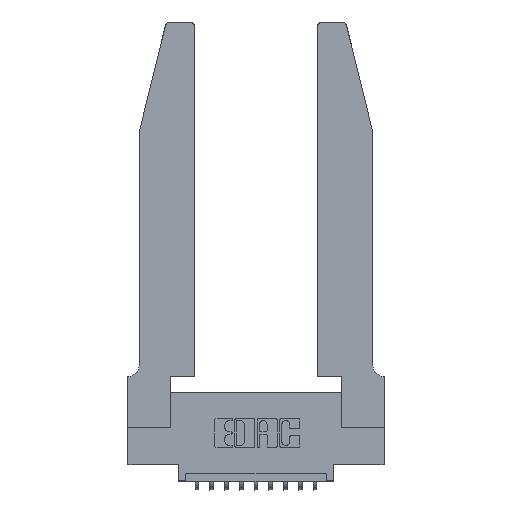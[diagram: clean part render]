
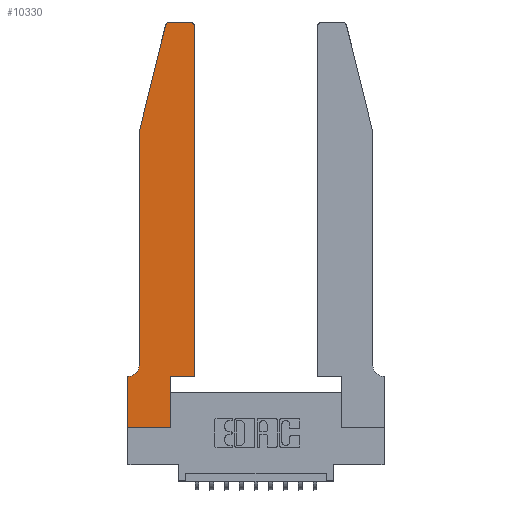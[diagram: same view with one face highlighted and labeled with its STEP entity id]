
A CAD part, top view. The second image highlights one B-rep face of the part: STEP entity #10330.
In plain terms, the highlighted planar face has unit normal (0, 0, 1).
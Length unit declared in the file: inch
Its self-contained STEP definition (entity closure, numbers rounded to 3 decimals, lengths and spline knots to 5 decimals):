
#149 = CARTESIAN_POINT ( 'NONE',  ( 0.25487, 2.72718, 0.37 ) ) ;
#305 = ORIENTED_EDGE ( 'NONE', *, *, #7473, .T. ) ;
#687 = DIRECTION ( 'NONE',  ( 0., 0., -1. ) ) ;
#851 = CARTESIAN_POINT ( 'NONE',  ( 0.4505, 2.72, 0.37 ) ) ;
#984 = EDGE_CURVE ( 'NONE', #15779, #5877, #7594, .T. ) ;
#1242 = ORIENTED_EDGE ( 'NONE', *, *, #15921, .T. ) ;
#1302 = VECTOR ( 'NONE', #8511, 39.37008 ) ;
#1312 = LINE ( 'NONE', #13618, #15610 ) ;
#1523 = CARTESIAN_POINT ( 'NONE',  ( 0.284, 2.72, 0.37 ) ) ;
#1672 = EDGE_CURVE ( 'NONE', #11569, #14212, #6824, .T. ) ;
#1750 = LINE ( 'NONE', #10745, #3556 ) ;
#1878 = CARTESIAN_POINT ( 'NONE',  ( 0.4205, 2.75, 0.37 ) ) ;
#1890 = EDGE_CURVE ( 'NONE', #8346, #9849, #11443, .T. ) ;
#2025 = CARTESIAN_POINT ( 'NONE',  ( 0., 0.35, 0.37 ) ) ;
#2319 = CARTESIAN_POINT ( 'NONE',  ( 0., 0., 0.37 ) ) ;
#2648 = VECTOR ( 'NONE', #5698, 39.37008 ) ;
#2650 = DIRECTION ( 'NONE',  ( 1., 0., 0. ) ) ;
#2751 = CIRCLE ( 'NONE', #11983, 0.07 ) ;
#2765 = DIRECTION ( 'NONE',  ( 0., 0., 1. ) ) ;
#3120 = LINE ( 'NONE', #12759, #15972 ) ;
#3165 = CIRCLE ( 'NONE', #11221, 0.03 ) ;
#3261 = DIRECTION ( 'NONE',  ( 0., 0., 1. ) ) ;
#3475 = CARTESIAN_POINT ( 'NONE',  ( 0.4505, 0.35, 0.37 ) ) ;
#3556 = VECTOR ( 'NONE', #6164, 39.37008 ) ;
#3619 = DIRECTION ( 'NONE',  ( -1., 0., 0. ) ) ;
#3727 = VECTOR ( 'NONE', #5262, 39.37008 ) ;
#4150 = AXIS2_PLACEMENT_3D ( 'NONE', #1523, #2765, #2650 ) ;
#5262 = DIRECTION ( 'NONE',  ( 0., -1., 0. ) ) ;
#5346 = ORIENTED_EDGE ( 'NONE', *, *, #984, .T. ) ;
#5553 = ORIENTED_EDGE ( 'NONE', *, *, #8800, .T. ) ;
#5608 = ORIENTED_EDGE ( 'NONE', *, *, #12032, .T. ) ;
#5698 = DIRECTION ( 'NONE',  ( 0., 1., 0. ) ) ;
#5722 = DIRECTION ( 'NONE',  ( 0., 0., 1. ) ) ;
#5734 = DIRECTION ( 'NONE',  ( -1., 0., 0. ) ) ;
#5860 = VECTOR ( 'NONE', #8008, 39.37008 ) ;
#5877 = VERTEX_POINT ( 'NONE', #15028 ) ;
#6164 = DIRECTION ( 'NONE',  ( 0., 1., 0. ) ) ;
#6606 = CARTESIAN_POINT ( 'NONE',  ( 0.2865, 0.35, 0.37 ) ) ;
#6824 = LINE ( 'NONE', #10971, #1302 ) ;
#6949 = DIRECTION ( 'NONE',  ( 1., 0., 0. ) ) ;
#6993 = VECTOR ( 'NONE', #15722, 39.37008 ) ;
#7071 = DIRECTION ( 'NONE',  ( -1., 0., 0. ) ) ;
#7079 = EDGE_LOOP ( 'NONE', ( #5608, #305, #15594, #7788, #9999, #5346, #1242, #8198, #13800, #7496, #5553, #13068 ) ) ;
#7351 = CARTESIAN_POINT ( 'NONE',  ( 0.0755, 2., 0.37 ) ) ;
#7473 = EDGE_CURVE ( 'NONE', #15290, #11569, #15079, .T. ) ;
#7496 = ORIENTED_EDGE ( 'NONE', *, *, #1890, .T. ) ;
#7594 = LINE ( 'NONE', #9414, #13465 ) ;
#7788 = ORIENTED_EDGE ( 'NONE', *, *, #12440, .T. ) ;
#7826 = CARTESIAN_POINT ( 'NONE',  ( 0.284, 2.75, 0.37 ) ) ;
#7921 = LINE ( 'NONE', #6606, #2648 ) ;
#8008 = DIRECTION ( 'NONE',  ( 1., 0., 0. ) ) ;
#8139 = CARTESIAN_POINT ( 'NONE',  ( 0.0055, 0.35, 0.37 ) ) ;
#8165 = PLANE ( 'NONE',  #14041 ) ;
#8198 = ORIENTED_EDGE ( 'NONE', *, *, #14521, .T. ) ;
#8346 = VERTEX_POINT ( 'NONE', #14619 ) ;
#8511 = DIRECTION ( 'NONE',  ( -0.239, -0.971, 0. ) ) ;
#8800 = EDGE_CURVE ( 'NONE', #9849, #13836, #1750, .T. ) ;
#9414 = CARTESIAN_POINT ( 'NONE',  ( 0.0755, 0.35, 0.37 ) ) ;
#9420 = DIRECTION ( 'NONE',  ( 1., 0., 0. ) ) ;
#9504 = EDGE_CURVE ( 'NONE', #13836, #12549, #3165, .T. ) ;
#9505 = VERTEX_POINT ( 'NONE', #15268 ) ;
#9849 = VERTEX_POINT ( 'NONE', #3475 ) ;
#9999 = ORIENTED_EDGE ( 'NONE', *, *, #14959, .T. ) ;
#10156 = CARTESIAN_POINT ( 'NONE',  ( 0.4205, 2.72, 0.37 ) ) ;
#10330 = ADVANCED_FACE ( 'NONE', ( #15618 ), #8165, .T. ) ;
#10689 = VERTEX_POINT ( 'NONE', #12643 ) ;
#10692 = LINE ( 'NONE', #13285, #6993 ) ;
#10745 = CARTESIAN_POINT ( 'NONE',  ( 0.4505, 0.35, 0.37 ) ) ;
#10748 = LINE ( 'NONE', #14633, #3727 ) ;
#10781 = CARTESIAN_POINT ( 'NONE',  ( 0.0055, 0.42, 0.37 ) ) ;
#10971 = CARTESIAN_POINT ( 'NONE',  ( 0.0755, 2., 0.37 ) ) ;
#11221 = AXIS2_PLACEMENT_3D ( 'NONE', #10156, #5722, #6949 ) ;
#11432 = DIRECTION ( 'NONE',  ( 0., -1., 0. ) ) ;
#11443 = LINE ( 'NONE', #11962, #5860 ) ;
#11569 = VERTEX_POINT ( 'NONE', #149 ) ;
#11962 = CARTESIAN_POINT ( 'NONE',  ( 0.4505, 0.35, 0.37 ) ) ;
#11983 = AXIS2_PLACEMENT_3D ( 'NONE', #10781, #687, #7071 ) ;
#12032 = EDGE_CURVE ( 'NONE', #12549, #15290, #1312, .T. ) ;
#12440 = EDGE_CURVE ( 'NONE', #14212, #9505, #3120, .T. ) ;
#12549 = VERTEX_POINT ( 'NONE', #1878 ) ;
#12643 = CARTESIAN_POINT ( 'NONE',  ( 0.2865, 0., 0.37 ) ) ;
#12759 = CARTESIAN_POINT ( 'NONE',  ( 0.0755, 2., 0.37 ) ) ;
#13068 = ORIENTED_EDGE ( 'NONE', *, *, #9504, .T. ) ;
#13285 = CARTESIAN_POINT ( 'NONE',  ( 0., 0., 0.37 ) ) ;
#13465 = VECTOR ( 'NONE', #5734, 39.37008 ) ;
#13618 = CARTESIAN_POINT ( 'NONE',  ( 0.2605, 2.75, 0.37 ) ) ;
#13800 = ORIENTED_EDGE ( 'NONE', *, *, #14028, .T. ) ;
#13836 = VERTEX_POINT ( 'NONE', #851 ) ;
#14028 = EDGE_CURVE ( 'NONE', #10689, #8346, #7921, .T. ) ;
#14041 = AXIS2_PLACEMENT_3D ( 'NONE', #2025, #3261, #9420 ) ;
#14188 = VERTEX_POINT ( 'NONE', #2319 ) ;
#14212 = VERTEX_POINT ( 'NONE', #7351 ) ;
#14521 = EDGE_CURVE ( 'NONE', #14188, #10689, #10692, .T. ) ;
#14619 = CARTESIAN_POINT ( 'NONE',  ( 0.2865, 0.35, 0.37 ) ) ;
#14633 = CARTESIAN_POINT ( 'NONE',  ( 0., 0., 0.37 ) ) ;
#14959 = EDGE_CURVE ( 'NONE', #9505, #15779, #2751, .T. ) ;
#15028 = CARTESIAN_POINT ( 'NONE',  ( 0., 0.35, 0.37 ) ) ;
#15079 = CIRCLE ( 'NONE', #4150, 0.03 ) ;
#15268 = CARTESIAN_POINT ( 'NONE',  ( 0.0755, 0.42, 0.37 ) ) ;
#15290 = VERTEX_POINT ( 'NONE', #7826 ) ;
#15594 = ORIENTED_EDGE ( 'NONE', *, *, #1672, .T. ) ;
#15610 = VECTOR ( 'NONE', #3619, 39.37008 ) ;
#15618 = FACE_OUTER_BOUND ( 'NONE', #7079, .T. ) ;
#15722 = DIRECTION ( 'NONE',  ( 1., 0., 0. ) ) ;
#15779 = VERTEX_POINT ( 'NONE', #8139 ) ;
#15921 = EDGE_CURVE ( 'NONE', #5877, #14188, #10748, .T. ) ;
#15972 = VECTOR ( 'NONE', #11432, 39.37008 ) ;
